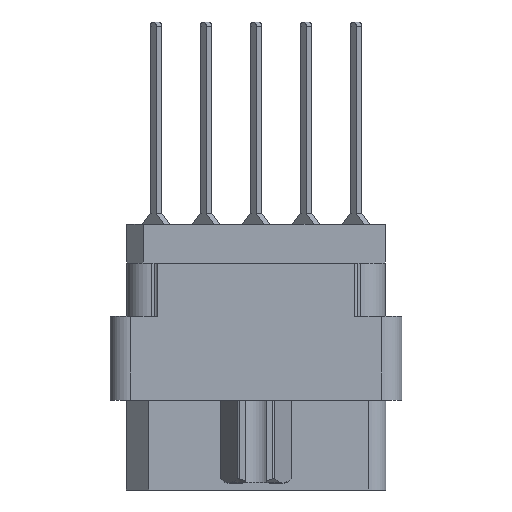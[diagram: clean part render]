
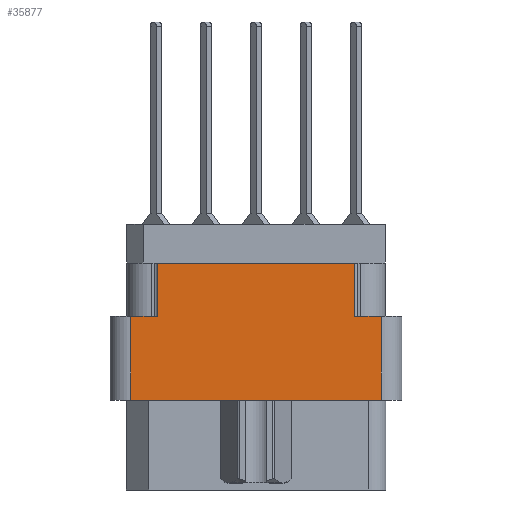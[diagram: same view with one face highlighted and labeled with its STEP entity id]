
A CAD part, left-side view. The second image highlights one B-rep face of the part: STEP entity #35877.
In plain terms, the highlighted planar face has unit normal (-1, 0, 0).
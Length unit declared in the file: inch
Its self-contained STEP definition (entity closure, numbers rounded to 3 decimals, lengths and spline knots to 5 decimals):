
#2065 = VERTEX_POINT ( 'NONE', #7141 ) ;
#2549 = CARTESIAN_POINT ( 'NONE',  ( -1., -0.296, -0.117 ) ) ;
#2696 = LINE ( 'NONE', #16608, #33258 ) ;
#4012 = LINE ( 'NONE', #38890, #21050 ) ;
#4269 = EDGE_CURVE ( 'NONE', #35524, #26663, #21269, .T. ) ;
#4466 = CARTESIAN_POINT ( 'NONE',  ( -1., 0.438, -0.117 ) ) ;
#5928 = EDGE_CURVE ( 'NONE', #6482, #2065, #4012, .T. ) ;
#6482 = VERTEX_POINT ( 'NONE', #38575 ) ;
#7141 = CARTESIAN_POINT ( 'NONE',  ( -1., -0.376, -0.277 ) ) ;
#7145 = VECTOR ( 'NONE', #33141, 39.37008 ) ;
#7191 = EDGE_CURVE ( 'NONE', #20615, #2065, #9476, .T. ) ;
#7247 = LINE ( 'NONE', #10446, #21114 ) ;
#8168 = CARTESIAN_POINT ( 'NONE',  ( -1., -0.296, -0.277 ) ) ;
#9476 = LINE ( 'NONE', #23417, #24719 ) ;
#10446 = CARTESIAN_POINT ( 'NONE',  ( -1., 0.376, -0.798 ) ) ;
#11687 = VECTOR ( 'NONE', #18358, 39.37008 ) ;
#12951 = EDGE_CURVE ( 'NONE', #26663, #23520, #38997, .T. ) ;
#14275 = DIRECTION ( 'NONE',  ( -1., 0., 0. ) ) ;
#15416 = VERTEX_POINT ( 'NONE', #2549 ) ;
#15822 = ORIENTED_EDGE ( 'NONE', *, *, #7191, .F. ) ;
#15929 = ORIENTED_EDGE ( 'NONE', *, *, #4269, .F. ) ;
#16608 = CARTESIAN_POINT ( 'NONE',  ( -1., -0.296, -0.277 ) ) ;
#16783 = DIRECTION ( 'NONE',  ( 0., -1., 0. ) ) ;
#17605 = DIRECTION ( 'NONE',  ( 0., -1., 0. ) ) ;
#17860 = EDGE_CURVE ( 'NONE', #23520, #15416, #35702, .T. ) ;
#17901 = DIRECTION ( 'NONE',  ( 0., 0., 1. ) ) ;
#18121 = ORIENTED_EDGE ( 'NONE', *, *, #17860, .F. ) ;
#18147 = DIRECTION ( 'NONE',  ( 0., 0., 1. ) ) ;
#18358 = DIRECTION ( 'NONE',  ( 0., -1., 0. ) ) ;
#20615 = VERTEX_POINT ( 'NONE', #8168 ) ;
#20741 = ORIENTED_EDGE ( 'NONE', *, *, #29349, .F. ) ;
#21050 = VECTOR ( 'NONE', #17901, 39.37008 ) ;
#21114 = VECTOR ( 'NONE', #41253, 39.37008 ) ;
#21269 = LINE ( 'NONE', #21959, #23160 ) ;
#21959 = CARTESIAN_POINT ( 'NONE',  ( -1., 0.438, -0.277 ) ) ;
#22877 = CARTESIAN_POINT ( 'NONE',  ( -1., 0.376, -0.277 ) ) ;
#23160 = VECTOR ( 'NONE', #17605, 39.37008 ) ;
#23417 = CARTESIAN_POINT ( 'NONE',  ( -1., -0.296, -0.277 ) ) ;
#23520 = VERTEX_POINT ( 'NONE', #37010 ) ;
#24719 = VECTOR ( 'NONE', #16783, 39.37008 ) ;
#25489 = EDGE_CURVE ( 'NONE', #20615, #15416, #2696, .T. ) ;
#26663 = VERTEX_POINT ( 'NONE', #41899 ) ;
#27324 = EDGE_CURVE ( 'NONE', #6482, #37773, #44333, .T. ) ;
#29349 = EDGE_CURVE ( 'NONE', #37773, #35524, #7247, .T. ) ;
#29800 = ORIENTED_EDGE ( 'NONE', *, *, #12951, .F. ) ;
#30073 = ORIENTED_EDGE ( 'NONE', *, *, #5928, .T. ) ;
#30866 = CARTESIAN_POINT ( 'NONE',  ( -1., 0.376, -0.529 ) ) ;
#33141 = DIRECTION ( 'NONE',  ( 0., 1., 0. ) ) ;
#33258 = VECTOR ( 'NONE', #44870, 39.37008 ) ;
#35253 = PLANE ( 'NONE',  #37903 ) ;
#35524 = VERTEX_POINT ( 'NONE', #22877 ) ;
#35702 = LINE ( 'NONE', #4466, #11687 ) ;
#35877 = ADVANCED_FACE ( 'NONE', ( #38459 ), #35253, .T. ) ;
#37010 = CARTESIAN_POINT ( 'NONE',  ( -1., 0.296, -0.117 ) ) ;
#37773 = VERTEX_POINT ( 'NONE', #30866 ) ;
#37903 = AXIS2_PLACEMENT_3D ( 'NONE', #38682, #14275, #18147 ) ;
#38212 = EDGE_LOOP ( 'NONE', ( #20741, #40570, #30073, #15822, #39618, #18121, #29800, #15929 ) ) ;
#38346 = VECTOR ( 'NONE', #38550, 39.37008 ) ;
#38459 = FACE_OUTER_BOUND ( 'NONE', #38212, .T. ) ;
#38550 = DIRECTION ( 'NONE',  ( 0., 0., 1. ) ) ;
#38575 = CARTESIAN_POINT ( 'NONE',  ( -1., -0.376, -0.529 ) ) ;
#38682 = CARTESIAN_POINT ( 'NONE',  ( -1., -0.376, -0.798 ) ) ;
#38890 = CARTESIAN_POINT ( 'NONE',  ( -1., -0.376, -0.798 ) ) ;
#38997 = LINE ( 'NONE', #42658, #38346 ) ;
#39618 = ORIENTED_EDGE ( 'NONE', *, *, #25489, .T. ) ;
#40570 = ORIENTED_EDGE ( 'NONE', *, *, #27324, .F. ) ;
#41253 = DIRECTION ( 'NONE',  ( 0., 0., 1. ) ) ;
#41899 = CARTESIAN_POINT ( 'NONE',  ( -1., 0.296, -0.277 ) ) ;
#42658 = CARTESIAN_POINT ( 'NONE',  ( -1., 0.296, -0.277 ) ) ;
#43650 = CARTESIAN_POINT ( 'NONE',  ( -1., -0.376, -0.529 ) ) ;
#44333 = LINE ( 'NONE', #43650, #7145 ) ;
#44870 = DIRECTION ( 'NONE',  ( 0., 0., 1. ) ) ;
